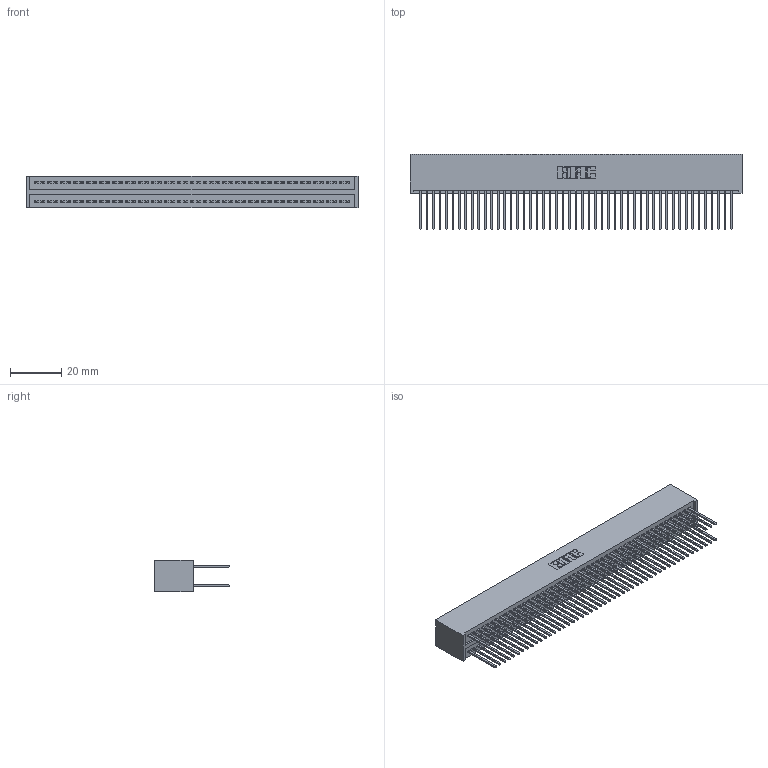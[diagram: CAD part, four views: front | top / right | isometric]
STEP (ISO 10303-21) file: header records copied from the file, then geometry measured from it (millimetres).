
FILE_DESCRIPTION (( 'STEP AP203' ), '1' );
FILE_NAME ('325-098-540-201.STEP', '2020-02-25T06:28:25', ( '' ), ( '' ), 'SwSTEP 2.0', 'SolidWorks 2016', '' );
FILE_SCHEMA (( 'CONFIG_CONTROL_DESIGN' ));
Length unit declared in the file: inch
Products named in the file (3): 325 Part_Lugless; 325-098-540-201; 325-292-001_325-293-140
Assembly tree (99 placements, depth 2):
  325-098-540-201
    325 Part_Lugless
    325-292-001_325-293-140  x98
Bounding box: 130.1 x 29.46 x 12.45 mm (x, y, z)
Volume: 17835.9 mm3; surface area: 24183.5 mm2
Topology: 99 solids, 99 shells, 5202 faces, 15477 edges, 10186 vertices
Faces by surface type: plane 3594, cylinder 1608
Entity records: 30359 total; most frequent: CARTESIAN_POINT 5022, ORIENTED_EDGE 4958, DIRECTION 4271, EDGE_CURVE 2479, LINE 2359, VECTOR 2359, VERTEX_POINT 1650, AXIS2_PLACEMENT_3D 956
